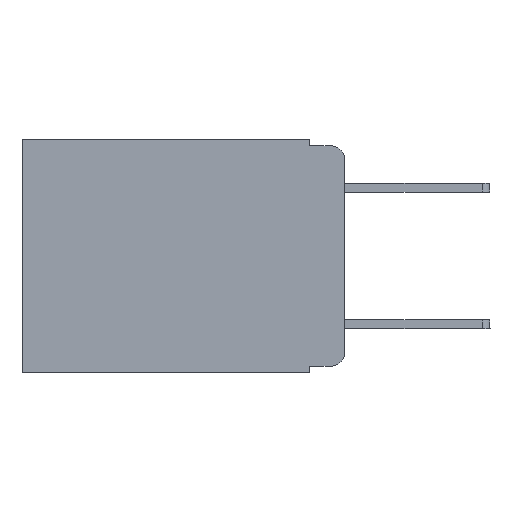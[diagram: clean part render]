
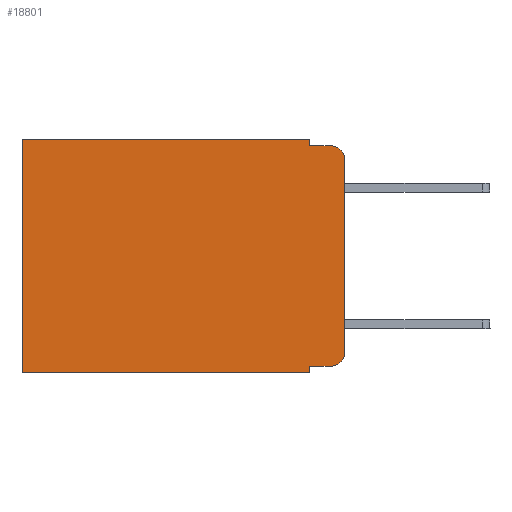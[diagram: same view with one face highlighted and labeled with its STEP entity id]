
A CAD part, left-side view. The second image highlights one B-rep face of the part: STEP entity #18801.
In plain terms, the highlighted planar face has unit normal (-1, 0, 0).
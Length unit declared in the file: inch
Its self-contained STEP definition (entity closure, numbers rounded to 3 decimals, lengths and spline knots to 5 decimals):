
#83 = DIRECTION ( 'NONE',  ( 0., 1., 0. ) ) ;
#131 = CARTESIAN_POINT ( 'NONE',  ( 0.298, 0.02, -0.313 ) ) ;
#151 = VECTOR ( 'NONE', #11426, 39.37008 ) ;
#536 = VERTEX_POINT ( 'NONE', #16596 ) ;
#1632 = FACE_OUTER_BOUND ( 'NONE', #14245, .T. ) ;
#1711 = AXIS2_PLACEMENT_3D ( 'NONE', #19048, #17031, #9639 ) ;
#2081 = VERTEX_POINT ( 'NONE', #10858 ) ;
#2342 = DIRECTION ( 'NONE',  ( 0., -1., 0. ) ) ;
#3547 = ORIENTED_EDGE ( 'NONE', *, *, #23369, .F. ) ;
#4229 = CARTESIAN_POINT ( 'NONE',  ( 0.298, 0.051, 0. ) ) ;
#4307 = EDGE_CURVE ( 'NONE', #7013, #4778, #13179, .T. ) ;
#4606 = VERTEX_POINT ( 'NONE', #8451 ) ;
#4778 = VERTEX_POINT ( 'NONE', #16832 ) ;
#4811 = AXIS2_PLACEMENT_3D ( 'NONE', #131, #8054, #15450 ) ;
#4892 = DIRECTION ( 'NONE',  ( 0., 0., -1. ) ) ;
#5883 = EDGE_CURVE ( 'NONE', #7342, #23061, #20926, .T. ) ;
#6101 = LINE ( 'NONE', #13747, #9531 ) ;
#6129 = ORIENTED_EDGE ( 'NONE', *, *, #9744, .T. ) ;
#6677 = ORIENTED_EDGE ( 'NONE', *, *, #22800, .F. ) ;
#6694 = ORIENTED_EDGE ( 'NONE', *, *, #4307, .F. ) ;
#6770 = LINE ( 'NONE', #20299, #10339 ) ;
#7013 = VERTEX_POINT ( 'NONE', #7277 ) ;
#7050 = CARTESIAN_POINT ( 'NONE',  ( 0.298, 0.051, -0.01 ) ) ;
#7277 = CARTESIAN_POINT ( 'NONE',  ( 0.298, 0.051, -0.343 ) ) ;
#7342 = VERTEX_POINT ( 'NONE', #16003 ) ;
#7591 = CIRCLE ( 'NONE', #4811, 0.02 ) ;
#7752 = CARTESIAN_POINT ( 'NONE',  ( 0.298, 0., 0. ) ) ;
#8020 = CARTESIAN_POINT ( 'NONE',  ( 0.298, 0.02, -0.01 ) ) ;
#8054 = DIRECTION ( 'NONE',  ( -1., 0., 0. ) ) ;
#8064 = ORIENTED_EDGE ( 'NONE', *, *, #5883, .F. ) ;
#8237 = LINE ( 'NONE', #4229, #24058 ) ;
#8243 = VERTEX_POINT ( 'NONE', #9951 ) ;
#8376 = EDGE_CURVE ( 'NONE', #7342, #22339, #14693, .T. ) ;
#8451 = CARTESIAN_POINT ( 'NONE',  ( 0.298, 0.051, 0. ) ) ;
#8464 = EDGE_CURVE ( 'NONE', #4606, #536, #16071, .T. ) ;
#8605 = CARTESIAN_POINT ( 'NONE',  ( 0.298, 0., 0. ) ) ;
#8704 = CARTESIAN_POINT ( 'NONE',  ( 0.298, 0.02, -0.333 ) ) ;
#9531 = VECTOR ( 'NONE', #2342, 39.37008 ) ;
#9639 = DIRECTION ( 'NONE',  ( 0., 0., -1. ) ) ;
#9744 = EDGE_CURVE ( 'NONE', #4606, #2081, #19161, .T. ) ;
#9951 = CARTESIAN_POINT ( 'NONE',  ( 0.298, 0.051, -0.333 ) ) ;
#10339 = VECTOR ( 'NONE', #4892, 39.37008 ) ;
#10806 = VECTOR ( 'NONE', #22591, 39.37008 ) ;
#10858 = CARTESIAN_POINT ( 'NONE',  ( 0.298, 0.473, 0. ) ) ;
#10925 = LINE ( 'NONE', #7050, #16853 ) ;
#11426 = DIRECTION ( 'NONE',  ( 0., 0., -1. ) ) ;
#12548 = ORIENTED_EDGE ( 'NONE', *, *, #8464, .F. ) ;
#12785 = EDGE_CURVE ( 'NONE', #8243, #21118, #6101, .T. ) ;
#13179 = LINE ( 'NONE', #20591, #10806 ) ;
#13747 = CARTESIAN_POINT ( 'NONE',  ( 0.298, 0.051, -0.333 ) ) ;
#13946 = VECTOR ( 'NONE', #22910, 39.37008 ) ;
#14245 = EDGE_LOOP ( 'NONE', ( #8064, #17599, #3547, #12548, #6129, #21682, #6694, #6677, #22684, #17603 ) ) ;
#14451 = DIRECTION ( 'NONE',  ( 0., 0., -1. ) ) ;
#14693 = CIRCLE ( 'NONE', #21837, 0.02 ) ;
#14717 = EDGE_CURVE ( 'NONE', #2081, #4778, #6770, .T. ) ;
#15450 = DIRECTION ( 'NONE',  ( 0., 0., -1. ) ) ;
#15747 = DIRECTION ( 'NONE',  ( 0., 0., -1. ) ) ;
#15893 = EDGE_CURVE ( 'NONE', #21118, #23061, #7591, .T. ) ;
#16003 = CARTESIAN_POINT ( 'NONE',  ( 0.298, 0., -0.03 ) ) ;
#16071 = LINE ( 'NONE', #23716, #151 ) ;
#16328 = CARTESIAN_POINT ( 'NONE',  ( 0.298, 0.02, -0.03 ) ) ;
#16451 = DIRECTION ( 'NONE',  ( -1., 0., 0. ) ) ;
#16596 = CARTESIAN_POINT ( 'NONE',  ( 0.298, 0.051, -0.01 ) ) ;
#16832 = CARTESIAN_POINT ( 'NONE',  ( 0.298, 0.473, -0.343 ) ) ;
#16853 = VECTOR ( 'NONE', #22214, 39.37008 ) ;
#17031 = DIRECTION ( 'NONE',  ( 1., 0., 0. ) ) ;
#17315 = CARTESIAN_POINT ( 'NONE',  ( 0.298, 0., -0.313 ) ) ;
#17599 = ORIENTED_EDGE ( 'NONE', *, *, #8376, .T. ) ;
#17603 = ORIENTED_EDGE ( 'NONE', *, *, #15893, .T. ) ;
#18801 = ADVANCED_FACE ( 'NONE', ( #1632 ), #20690, .F. ) ;
#19048 = CARTESIAN_POINT ( 'NONE',  ( 0.298, 0., 0. ) ) ;
#19161 = LINE ( 'NONE', #8605, #23022 ) ;
#20299 = CARTESIAN_POINT ( 'NONE',  ( 0.298, 0.473, 0. ) ) ;
#20591 = CARTESIAN_POINT ( 'NONE',  ( 0.298, 0., -0.343 ) ) ;
#20690 = PLANE ( 'NONE',  #1711 ) ;
#20926 = LINE ( 'NONE', #7752, #13946 ) ;
#21118 = VERTEX_POINT ( 'NONE', #8704 ) ;
#21682 = ORIENTED_EDGE ( 'NONE', *, *, #14717, .T. ) ;
#21837 = AXIS2_PLACEMENT_3D ( 'NONE', #16328, #16451, #14451 ) ;
#22214 = DIRECTION ( 'NONE',  ( 0., -1., 0. ) ) ;
#22339 = VERTEX_POINT ( 'NONE', #8020 ) ;
#22591 = DIRECTION ( 'NONE',  ( 0., 1., 0. ) ) ;
#22684 = ORIENTED_EDGE ( 'NONE', *, *, #12785, .T. ) ;
#22800 = EDGE_CURVE ( 'NONE', #8243, #7013, #8237, .T. ) ;
#22910 = DIRECTION ( 'NONE',  ( 0., 0., -1. ) ) ;
#23022 = VECTOR ( 'NONE', #83, 39.37008 ) ;
#23061 = VERTEX_POINT ( 'NONE', #17315 ) ;
#23369 = EDGE_CURVE ( 'NONE', #536, #22339, #10925, .T. ) ;
#23716 = CARTESIAN_POINT ( 'NONE',  ( 0.298, 0.051, 0. ) ) ;
#24058 = VECTOR ( 'NONE', #15747, 39.37008 ) ;
